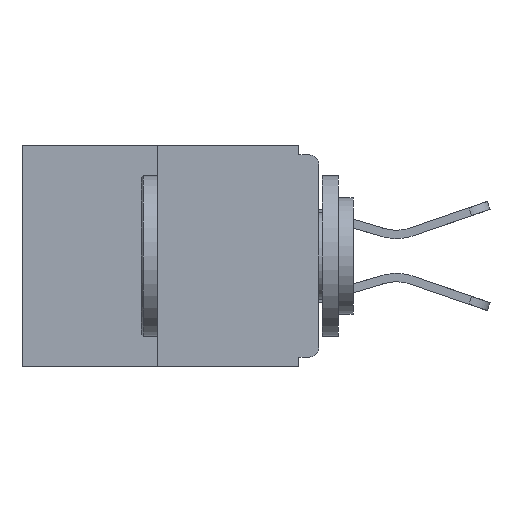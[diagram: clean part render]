
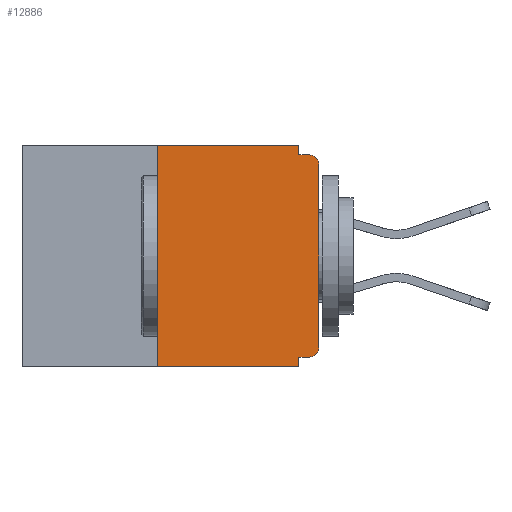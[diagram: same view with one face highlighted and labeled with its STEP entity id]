
A CAD part, left-side view. The second image highlights one B-rep face of the part: STEP entity #12886.
In plain terms, the highlighted planar face has unit normal (-1, 0, 0).
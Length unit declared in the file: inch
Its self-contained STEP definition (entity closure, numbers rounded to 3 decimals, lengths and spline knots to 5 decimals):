
#62 = CARTESIAN_POINT ( 'NONE',  ( 0., 0., -0.328 ) ) ;
#135 = CARTESIAN_POINT ( 'NONE',  ( 0., 0., 0. ) ) ;
#433 = EDGE_CURVE ( 'NONE', #5962, #891, #4055, .T. ) ;
#568 = VERTEX_POINT ( 'NONE', #16825 ) ;
#891 = VERTEX_POINT ( 'NONE', #19266 ) ;
#950 = EDGE_CURVE ( 'NONE', #3159, #5962, #10330, .T. ) ;
#1018 = DIRECTION ( 'NONE',  ( -1., 0., 0. ) ) ;
#1348 = AXIS2_PLACEMENT_3D ( 'NONE', #4170, #16002, #14748 ) ;
#2050 = ORIENTED_EDGE ( 'NONE', *, *, #3711, .T. ) ;
#2342 = DIRECTION ( 'NONE',  ( 0., 0., 1. ) ) ;
#2370 = CARTESIAN_POINT ( 'NONE',  ( 0., 0.25, -0.343 ) ) ;
#2650 = CARTESIAN_POINT ( 'NONE',  ( 0., 0.015, -0.03 ) ) ;
#2765 = CARTESIAN_POINT ( 'NONE',  ( 0., 0.031, -0.015 ) ) ;
#2800 = EDGE_LOOP ( 'NONE', ( #8415, #9160, #11086, #17737, #4573, #2050, #11349, #18171, #18083, #17023 ) ) ;
#3159 = VERTEX_POINT ( 'NONE', #15422 ) ;
#3580 = DIRECTION ( 'NONE',  ( 0., -1., 0. ) ) ;
#3711 = EDGE_CURVE ( 'NONE', #3159, #568, #9519, .T. ) ;
#4055 = LINE ( 'NONE', #11602, #14994 ) ;
#4170 = CARTESIAN_POINT ( 'NONE',  ( 0., 0.015, -0.313 ) ) ;
#4241 = EDGE_CURVE ( 'NONE', #15393, #7229, #16036, .T. ) ;
#4444 = LINE ( 'NONE', #16977, #8582 ) ;
#4491 = DIRECTION ( 'NONE',  ( 0., 0., -1. ) ) ;
#4573 = ORIENTED_EDGE ( 'NONE', *, *, #950, .F. ) ;
#4779 = VERTEX_POINT ( 'NONE', #8727 ) ;
#5962 = VERTEX_POINT ( 'NONE', #14995 ) ;
#6326 = DIRECTION ( 'NONE',  ( 0., -1., 0. ) ) ;
#6358 = CARTESIAN_POINT ( 'NONE',  ( 0., 0.031, 0. ) ) ;
#6812 = AXIS2_PLACEMENT_3D ( 'NONE', #2650, #1018, #12888 ) ;
#7229 = VERTEX_POINT ( 'NONE', #16982 ) ;
#7446 = CARTESIAN_POINT ( 'NONE',  ( 0., 0.46, 0. ) ) ;
#7630 = CARTESIAN_POINT ( 'NONE',  ( 0., 0.031, 0. ) ) ;
#8032 = VECTOR ( 'NONE', #12416, 39.37008 ) ;
#8415 = ORIENTED_EDGE ( 'NONE', *, *, #16922, .F. ) ;
#8476 = EDGE_CURVE ( 'NONE', #13722, #9673, #16902, .T. ) ;
#8582 = VECTOR ( 'NONE', #2342, 39.37008 ) ;
#8727 = CARTESIAN_POINT ( 'NONE',  ( 0., 0.25, 0. ) ) ;
#8941 = DIRECTION ( 'NONE',  ( 1., 0., 0. ) ) ;
#9096 = DIRECTION ( 'NONE',  ( 0., 0., 1. ) ) ;
#9160 = ORIENTED_EDGE ( 'NONE', *, *, #11051, .F. ) ;
#9328 = AXIS2_PLACEMENT_3D ( 'NONE', #7446, #8941, #4491 ) ;
#9519 = CIRCLE ( 'NONE', #1348, 0.015 ) ;
#9603 = VECTOR ( 'NONE', #13469, 39.37008 ) ;
#9673 = VERTEX_POINT ( 'NONE', #2765 ) ;
#9987 = CARTESIAN_POINT ( 'NONE',  ( 0., 0.46, -0.343 ) ) ;
#10217 = EDGE_CURVE ( 'NONE', #9673, #7229, #10310, .T. ) ;
#10310 = LINE ( 'NONE', #16894, #17296 ) ;
#10330 = LINE ( 'NONE', #62, #9603 ) ;
#11051 = EDGE_CURVE ( 'NONE', #13144, #4779, #4444, .T. ) ;
#11086 = ORIENTED_EDGE ( 'NONE', *, *, #16573, .T. ) ;
#11349 = ORIENTED_EDGE ( 'NONE', *, *, #14015, .T. ) ;
#11602 = CARTESIAN_POINT ( 'NONE',  ( 0., 0.031, -0.343 ) ) ;
#11771 = VECTOR ( 'NONE', #3580, 39.37008 ) ;
#12093 = LINE ( 'NONE', #135, #14413 ) ;
#12152 = FACE_OUTER_BOUND ( 'NONE', #2800, .T. ) ;
#12416 = DIRECTION ( 'NONE',  ( 0., 0., -1. ) ) ;
#12495 = LINE ( 'NONE', #9987, #19036 ) ;
#12886 = ADVANCED_FACE ( 'NONE', ( #12152 ), #16432, .F. ) ;
#12888 = DIRECTION ( 'NONE',  ( 0., 0., -1. ) ) ;
#13144 = VERTEX_POINT ( 'NONE', #2370 ) ;
#13469 = DIRECTION ( 'NONE',  ( 0., 1., 0. ) ) ;
#13598 = CARTESIAN_POINT ( 'NONE',  ( 0., 0., -0.03 ) ) ;
#13722 = VERTEX_POINT ( 'NONE', #7630 ) ;
#13970 = CARTESIAN_POINT ( 'NONE',  ( 0., 0.46, 0. ) ) ;
#14015 = EDGE_CURVE ( 'NONE', #568, #15393, #12093, .T. ) ;
#14413 = VECTOR ( 'NONE', #9096, 39.37008 ) ;
#14748 = DIRECTION ( 'NONE',  ( 0., 0., -1. ) ) ;
#14994 = VECTOR ( 'NONE', #19197, 39.37008 ) ;
#14995 = CARTESIAN_POINT ( 'NONE',  ( 0., 0.031, -0.328 ) ) ;
#15393 = VERTEX_POINT ( 'NONE', #13598 ) ;
#15422 = CARTESIAN_POINT ( 'NONE',  ( 0., 0.015, -0.328 ) ) ;
#16002 = DIRECTION ( 'NONE',  ( -1., 0., 0. ) ) ;
#16036 = CIRCLE ( 'NONE', #6812, 0.015 ) ;
#16432 = PLANE ( 'NONE',  #9328 ) ;
#16573 = EDGE_CURVE ( 'NONE', #13144, #891, #12495, .T. ) ;
#16825 = CARTESIAN_POINT ( 'NONE',  ( 0., 0., -0.313 ) ) ;
#16894 = CARTESIAN_POINT ( 'NONE',  ( 0., 0., -0.015 ) ) ;
#16902 = LINE ( 'NONE', #6358, #8032 ) ;
#16922 = EDGE_CURVE ( 'NONE', #4779, #13722, #19272, .T. ) ;
#16977 = CARTESIAN_POINT ( 'NONE',  ( 0., 0.25, 0. ) ) ;
#16982 = CARTESIAN_POINT ( 'NONE',  ( 0., 0.015, -0.015 ) ) ;
#17023 = ORIENTED_EDGE ( 'NONE', *, *, #8476, .F. ) ;
#17296 = VECTOR ( 'NONE', #6326, 39.37008 ) ;
#17420 = DIRECTION ( 'NONE',  ( 0., -1., 0. ) ) ;
#17737 = ORIENTED_EDGE ( 'NONE', *, *, #433, .F. ) ;
#18083 = ORIENTED_EDGE ( 'NONE', *, *, #10217, .F. ) ;
#18171 = ORIENTED_EDGE ( 'NONE', *, *, #4241, .T. ) ;
#19036 = VECTOR ( 'NONE', #17420, 39.37008 ) ;
#19197 = DIRECTION ( 'NONE',  ( 0., 0., -1. ) ) ;
#19266 = CARTESIAN_POINT ( 'NONE',  ( 0., 0.031, -0.343 ) ) ;
#19272 = LINE ( 'NONE', #13970, #11771 ) ;
